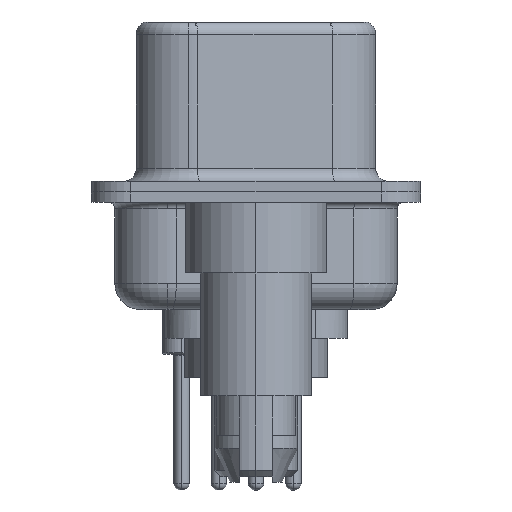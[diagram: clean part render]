
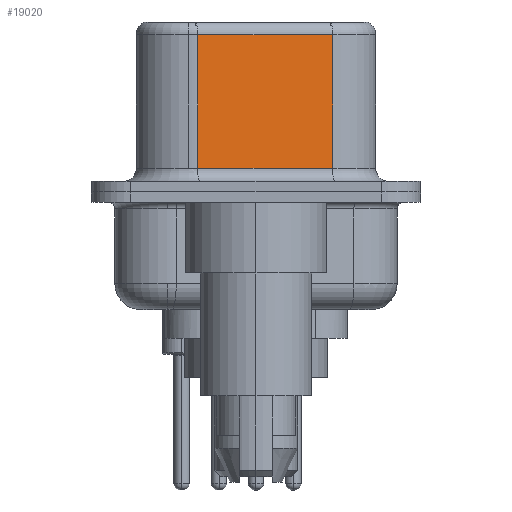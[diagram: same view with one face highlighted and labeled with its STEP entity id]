
A CAD part, left-side view. The second image highlights one B-rep face of the part: STEP entity #19020.
In plain terms, the highlighted planar face has unit normal (-0.985, -0.174, 0).
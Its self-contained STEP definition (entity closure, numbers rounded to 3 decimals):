
#1263 = ORIENTED_EDGE ( 'NONE', *, *, #19377, .F. ) ;
#1384 = VERTEX_POINT ( 'NONE', #16697 ) ;
#1413 = EDGE_CURVE ( 'NONE', #1384, #7343, #2788, .T. ) ;
#1753 = ORIENTED_EDGE ( 'NONE', *, *, #17583, .T. ) ;
#2105 = ORIENTED_EDGE ( 'NONE', *, *, #18306, .T. ) ;
#2271 = VECTOR ( 'NONE', #21174, 1000. ) ;
#2788 = LINE ( 'NONE', #9253, #2271 ) ;
#3076 = CARTESIAN_POINT ( 'NONE',  ( 4.58, -2.927, 6.52 ) ) ;
#3564 = VECTOR ( 'NONE', #18235, 1000. ) ;
#4260 = VECTOR ( 'NONE', #7220, 1000. ) ;
#5579 = CARTESIAN_POINT ( 'NONE',  ( 4.58, -2.927, 6.52 ) ) ;
#6075 = VERTEX_POINT ( 'NONE', #14409 ) ;
#6384 = PLANE ( 'NONE',  #11199 ) ;
#6836 = LINE ( 'NONE', #16590, #3564 ) ;
#7220 = DIRECTION ( 'NONE',  ( 0., 0., -1. ) ) ;
#7343 = VERTEX_POINT ( 'NONE', #20268 ) ;
#8040 = DIRECTION ( 'NONE',  ( -0.174, 0.985, 0. ) ) ;
#8092 = VECTOR ( 'NONE', #8681, 1000. ) ;
#8681 = DIRECTION ( 'NONE',  ( 0., 0., -1. ) ) ;
#8758 = EDGE_LOOP ( 'NONE', ( #1263, #1753, #2105, #12167 ) ) ;
#9253 = CARTESIAN_POINT ( 'NONE',  ( 4.58, -2.927, 0.9 ) ) ;
#11118 = CARTESIAN_POINT ( 'NONE',  ( 3.67, 2.233, 6.02 ) ) ;
#11199 = AXIS2_PLACEMENT_3D ( 'NONE', #3076, #17853, #8040 ) ;
#11621 = VERTEX_POINT ( 'NONE', #11118 ) ;
#12167 = ORIENTED_EDGE ( 'NONE', *, *, #1413, .T. ) ;
#12929 = LINE ( 'NONE', #5579, #4260 ) ;
#14409 = CARTESIAN_POINT ( 'NONE',  ( 4.58, -2.927, 6.02 ) ) ;
#16590 = CARTESIAN_POINT ( 'NONE',  ( 4.58, -2.927, 6.02 ) ) ;
#16697 = CARTESIAN_POINT ( 'NONE',  ( 3.67, 2.233, 0.9 ) ) ;
#16793 = LINE ( 'NONE', #18508, #8092 ) ;
#17583 = EDGE_CURVE ( 'NONE', #6075, #11621, #6836, .T. ) ;
#17853 = DIRECTION ( 'NONE',  ( 0.985, 0.174, 0. ) ) ;
#18235 = DIRECTION ( 'NONE',  ( -0.174, 0.985, 0. ) ) ;
#18306 = EDGE_CURVE ( 'NONE', #11621, #1384, #16793, .T. ) ;
#18508 = CARTESIAN_POINT ( 'NONE',  ( 3.67, 2.233, 6.52 ) ) ;
#19020 = ADVANCED_FACE ( 'NONE', ( #20695 ), #6384, .F. ) ;
#19377 = EDGE_CURVE ( 'NONE', #6075, #7343, #12929, .T. ) ;
#20268 = CARTESIAN_POINT ( 'NONE',  ( 4.58, -2.927, 0.9 ) ) ;
#20695 = FACE_OUTER_BOUND ( 'NONE', #8758, .T. ) ;
#21174 = DIRECTION ( 'NONE',  ( 0.174, -0.985, 0. ) ) ;
